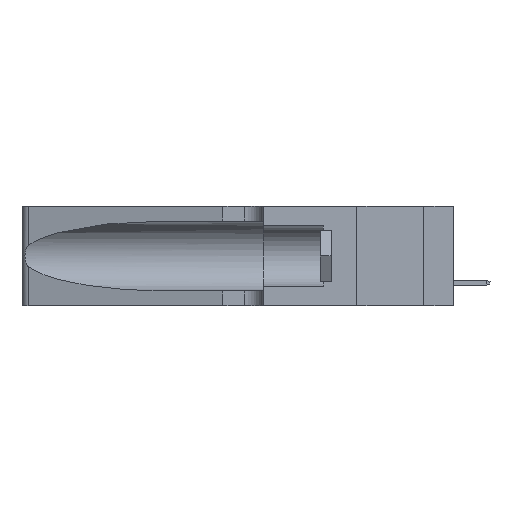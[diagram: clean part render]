
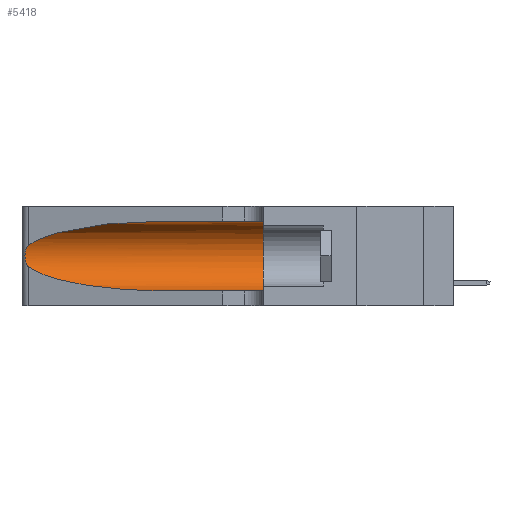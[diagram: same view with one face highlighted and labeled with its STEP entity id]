
A CAD part, left-side view. The second image highlights one B-rep face of the part: STEP entity #5418.
In plain terms, the highlighted cylindrical face has radius 3.308 mm (diameter 6.617 mm), a partial arc.
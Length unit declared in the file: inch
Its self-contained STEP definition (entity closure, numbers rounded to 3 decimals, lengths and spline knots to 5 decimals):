
#412 = CARTESIAN_POINT ( 'NONE',  ( 0.25487, 1.22718, 0.14631 ) ) ;
#782 = CARTESIAN_POINT ( 'NONE',  ( 0.1305, 0.35, 0.05475 ) ) ;
#892 = EDGE_CURVE ( 'NONE', #8655, #9955, #17333, .T. ) ;
#974 = CARTESIAN_POINT ( 'NONE',  ( 0.25487, 1.22718, 0.14631 ) ) ;
#1197 = DIRECTION ( 'NONE',  ( 0., 0., -1. ) ) ;
#2071 = DIRECTION ( 'NONE',  ( 0., -1., 0. ) ) ;
#2245 = CARTESIAN_POINT ( 'NONE',  ( 0.25787, 1.23484, 0.2124 ) ) ;
#2336 = CARTESIAN_POINT ( 'NONE',  ( 0.25856, 1.23593, 0.16098 ) ) ;
#2377 = CYLINDRICAL_SURFACE ( 'NONE', #3365, 0.13025 ) ;
#2515 = CARTESIAN_POINT ( 'NONE',  ( 0.1305, 0.72297, 0.31525 ) ) ;
#2608 = LINE ( 'NONE', #15264, #17623 ) ;
#3365 = AXIS2_PLACEMENT_3D ( 'NONE', #6376, #11932, #1197 ) ;
#3598 = CARTESIAN_POINT ( 'NONE',  ( 0.25639, 1.23184, 0.21858 ) ) ;
#3726 = FACE_OUTER_BOUND ( 'NONE', #12383, .T. ) ;
#3770 = CARTESIAN_POINT ( 'NONE',  ( 0.25854, 1.2359, 0.20912 ) ) ;
#4496 = CARTESIAN_POINT ( 'NONE',  ( 0.18966, 0.96281, 0.05475 ) ) ;
#4570 = DIRECTION ( 'NONE',  ( 0., 0., 1. ) ) ;
#4595 = VECTOR ( 'NONE', #14818, 39.37008 ) ;
#5228 = CARTESIAN_POINT ( 'NONE',  ( 0.26075, 1.23896, 0.19203 ) ) ;
#5418 = ADVANCED_FACE ( 'NONE', ( #3726 ), #2377, .F. ) ;
#6206 = ORIENTED_EDGE ( 'NONE', *, *, #15209, .T. ) ;
#6376 = CARTESIAN_POINT ( 'NONE',  ( 0.1305, 1.61858, 0.185 ) ) ;
#6589 = CARTESIAN_POINT ( 'NONE',  ( 0.26018, 1.23835, 0.19895 ) ) ;
#7084 = EDGE_CURVE ( 'NONE', #14619, #15431, #9534, .T. ) ;
#7380 = AXIS2_PLACEMENT_3D ( 'NONE', #11399, #14233, #4570 ) ;
#7388 = CARTESIAN_POINT ( 'NONE',  ( 0.2373, 1.15595, 0.08982 ) ) ;
#7702 = EDGE_CURVE ( 'NONE', #9955, #8324, #15425, .T. ) ;
#7791 = CARTESIAN_POINT ( 'NONE',  ( 0.26017, 1.23833, 0.17102 ) ) ;
#7831 = ORIENTED_EDGE ( 'NONE', *, *, #892, .T. ) ;
#7880 = CARTESIAN_POINT ( 'NONE',  ( 0.25555, 1.22993, 0.14849 ) ) ;
#8324 = VERTEX_POINT ( 'NONE', #11826 ) ;
#8655 = VERTEX_POINT ( 'NONE', #13187 ) ;
#9186 =( BOUNDED_CURVE ( )  B_SPLINE_CURVE ( 3, ( #2515, #9277, #11989, #17771 ),
 .UNSPECIFIED., .F., .F. ) 
 B_SPLINE_CURVE_WITH_KNOTS ( ( 4, 4 ),
 ( 1.5708, 2.84003 ),
 .UNSPECIFIED. ) 
 CURVE ( )  GEOMETRIC_REPRESENTATION_ITEM ( )  RATIONAL_B_SPLINE_CURVE ( ( 1., 0.87, 0.87, 1. ) ) 
 REPRESENTATION_ITEM ( '' )  );
#9265 = CARTESIAN_POINT ( 'NONE',  ( 0.25639, 1.23186, 0.15144 ) ) ;
#9277 = CARTESIAN_POINT ( 'NONE',  ( 0.18966, 0.96281, 0.31525 ) ) ;
#9396 = ORIENTED_EDGE ( 'NONE', *, *, #7084, .F. ) ;
#9439 = CARTESIAN_POINT ( 'NONE',  ( 0.25555, 1.22994, 0.2215 ) ) ;
#9534 = LINE ( 'NONE', #12163, #4595 ) ;
#9872 = ORIENTED_EDGE ( 'NONE', *, *, #12905, .F. ) ;
#9955 = VERTEX_POINT ( 'NONE', #16801 ) ;
#11399 = CARTESIAN_POINT ( 'NONE',  ( 0.1305, 0.35, 0.185 ) ) ;
#11826 = CARTESIAN_POINT ( 'NONE',  ( 0.1305, 0.72297, 0.05475 ) ) ;
#11932 = DIRECTION ( 'NONE',  ( 0., -1., 0. ) ) ;
#11943 = ORIENTED_EDGE ( 'NONE', *, *, #16328, .T. ) ;
#11989 = CARTESIAN_POINT ( 'NONE',  ( 0.2373, 1.15595, 0.28018 ) ) ;
#12146 = CARTESIAN_POINT ( 'NONE',  ( 0.25789, 1.23486, 0.15765 ) ) ;
#12163 = CARTESIAN_POINT ( 'NONE',  ( 0.1305, 1.61858, 0.31525 ) ) ;
#12383 = EDGE_LOOP ( 'NONE', ( #6206, #7831, #17387, #11943, #9872, #9396 ) ) ;
#12905 = EDGE_CURVE ( 'NONE', #15431, #15765, #15239, .T. ) ;
#13187 = CARTESIAN_POINT ( 'NONE',  ( 0.25487, 1.22718, 0.22369 ) ) ;
#14233 = DIRECTION ( 'NONE',  ( 0., 1., 0. ) ) ;
#14363 = CARTESIAN_POINT ( 'NONE',  ( 0.1305, 0.72297, 0.31525 ) ) ;
#14619 = VERTEX_POINT ( 'NONE', #14363 ) ;
#14818 = DIRECTION ( 'NONE',  ( 0., -1., 0. ) ) ;
#14888 = CARTESIAN_POINT ( 'NONE',  ( 0.1305, 0.35, 0.31525 ) ) ;
#15209 = EDGE_CURVE ( 'NONE', #14619, #8655, #9186, .T. ) ;
#15239 = CIRCLE ( 'NONE', #7380, 0.13025 ) ;
#15264 = CARTESIAN_POINT ( 'NONE',  ( 0.1305, 1.61858, 0.05475 ) ) ;
#15425 =( BOUNDED_CURVE ( )  B_SPLINE_CURVE ( 3, ( #412, #7388, #4496, #15679 ),
 .UNSPECIFIED., .F., .T. ) 
 B_SPLINE_CURVE_WITH_KNOTS ( ( 4, 4 ),
 ( 3.44316, 4.71239 ),
 .UNSPECIFIED. ) 
 CURVE ( )  GEOMETRIC_REPRESENTATION_ITEM ( )  RATIONAL_B_SPLINE_CURVE ( ( 1., 0.87, 0.87, 1. ) ) 
 REPRESENTATION_ITEM ( '' )  );
#15431 = VERTEX_POINT ( 'NONE', #14888 ) ;
#15679 = CARTESIAN_POINT ( 'NONE',  ( 0.1305, 0.72297, 0.05475 ) ) ;
#15765 = VERTEX_POINT ( 'NONE', #782 ) ;
#16236 = CARTESIAN_POINT ( 'NONE',  ( 0.26075, 1.23896, 0.178 ) ) ;
#16328 = EDGE_CURVE ( 'NONE', #8324, #15765, #2608, .T. ) ;
#16801 = CARTESIAN_POINT ( 'NONE',  ( 0.25487, 1.22718, 0.14631 ) ) ;
#17333 = B_SPLINE_CURVE_WITH_KNOTS ( 'NONE', 3,
 ( #17674, #9439, #3598, #2245, #3770, #6589, #5228, #16236, #7791, #2336, #12146, #9265, #7880, #974 ),
 .UNSPECIFIED., .F., .F.,
 ( 4, 2, 2, 2, 2, 2, 4 ),
 ( 0., 0.00027, 0.00053, 0.00107, 0.0016, 0.00187, 0.00214 ),
 .UNSPECIFIED. ) ;
#17387 = ORIENTED_EDGE ( 'NONE', *, *, #7702, .T. ) ;
#17623 = VECTOR ( 'NONE', #2071, 39.37008 ) ;
#17674 = CARTESIAN_POINT ( 'NONE',  ( 0.25487, 1.22718, 0.22369 ) ) ;
#17771 = CARTESIAN_POINT ( 'NONE',  ( 0.25487, 1.22718, 0.22369 ) ) ;
